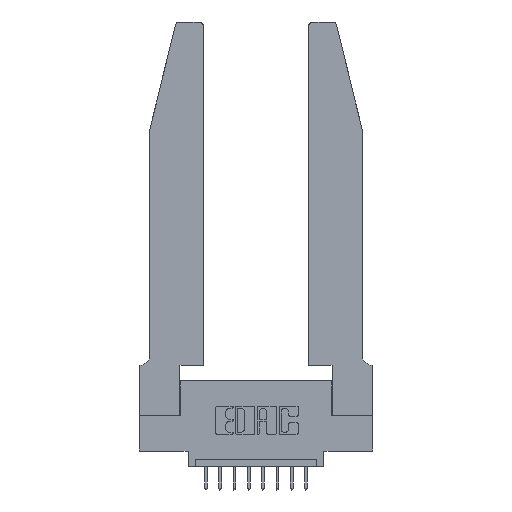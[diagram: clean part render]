
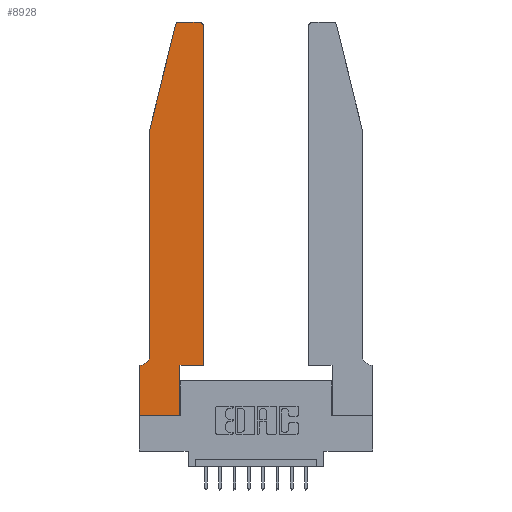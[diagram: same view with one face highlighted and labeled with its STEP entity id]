
A CAD part, top view. The second image highlights one B-rep face of the part: STEP entity #8928.
In plain terms, the highlighted planar face has unit normal (0, 0, 1).
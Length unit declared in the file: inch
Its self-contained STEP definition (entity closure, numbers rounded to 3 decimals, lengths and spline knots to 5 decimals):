
#104 = PLANE ( 'NONE',  #12794 ) ;
#188 = EDGE_CURVE ( 'NONE', #14460, #11975, #10427, .T. ) ;
#436 = EDGE_LOOP ( 'NONE', ( #5661, #9876, #15325, #4013, #3837, #6668, #12609, #13823, #14365, #1613, #8005, #14443 ) ) ;
#572 = VERTEX_POINT ( 'NONE', #828 ) ;
#698 = CARTESIAN_POINT ( 'NONE',  ( 0.4505, 0.35, 0.37 ) ) ;
#756 = DIRECTION ( 'NONE',  ( -1., 0., 0. ) ) ;
#828 = CARTESIAN_POINT ( 'NONE',  ( 0.4505, 0.35, 0.37 ) ) ;
#941 = AXIS2_PLACEMENT_3D ( 'NONE', #3066, #14900, #7694 ) ;
#1211 = CARTESIAN_POINT ( 'NONE',  ( 0., 0., 0.37 ) ) ;
#1532 = CARTESIAN_POINT ( 'NONE',  ( 0.2865, 0.35, 0.37 ) ) ;
#1562 = CARTESIAN_POINT ( 'NONE',  ( 0.0755, 0.42, 0.37 ) ) ;
#1613 = ORIENTED_EDGE ( 'NONE', *, *, #8762, .T. ) ;
#1659 = DIRECTION ( 'NONE',  ( -1., 0., 0. ) ) ;
#1669 = CARTESIAN_POINT ( 'NONE',  ( 0.0755, 0.35, 0.37 ) ) ;
#1812 = DIRECTION ( 'NONE',  ( 1., 0., 0. ) ) ;
#1844 = LINE ( 'NONE', #698, #15187 ) ;
#1859 = DIRECTION ( 'NONE',  ( 0., 1., 0. ) ) ;
#1860 = LINE ( 'NONE', #6751, #10148 ) ;
#1892 = DIRECTION ( 'NONE',  ( 0., 0., -1. ) ) ;
#1962 = CARTESIAN_POINT ( 'NONE',  ( 0.2865, 0.35, 0.37 ) ) ;
#2010 = DIRECTION ( 'NONE',  ( 0., -1., 0. ) ) ;
#2581 = DIRECTION ( 'NONE',  ( 1., 0., 0. ) ) ;
#2660 = EDGE_CURVE ( 'NONE', #9801, #9125, #14091, .T. ) ;
#3066 = CARTESIAN_POINT ( 'NONE',  ( 0.284, 2.72, 0.37 ) ) ;
#3127 = CARTESIAN_POINT ( 'NONE',  ( 0.2605, 2.75, 0.37 ) ) ;
#3391 = DIRECTION ( 'NONE',  ( 0., 0., 1. ) ) ;
#3406 = LINE ( 'NONE', #1962, #6804 ) ;
#3455 = CIRCLE ( 'NONE', #941, 0.03 ) ;
#3666 = CARTESIAN_POINT ( 'NONE',  ( 0.4505, 2.72, 0.37 ) ) ;
#3747 = CARTESIAN_POINT ( 'NONE',  ( 0.4205, 2.75, 0.37 ) ) ;
#3837 = ORIENTED_EDGE ( 'NONE', *, *, #2660, .T. ) ;
#4013 = ORIENTED_EDGE ( 'NONE', *, *, #11783, .T. ) ;
#4332 = DIRECTION ( 'NONE',  ( -0.239, -0.971, 0. ) ) ;
#4358 = VECTOR ( 'NONE', #1812, 39.37008 ) ;
#5359 = VERTEX_POINT ( 'NONE', #12533 ) ;
#5596 = EDGE_CURVE ( 'NONE', #13138, #5359, #3455, .T. ) ;
#5661 = ORIENTED_EDGE ( 'NONE', *, *, #14688, .T. ) ;
#5752 = CARTESIAN_POINT ( 'NONE',  ( 0.4205, 2.72, 0.37 ) ) ;
#5823 = CARTESIAN_POINT ( 'NONE',  ( 0.0755, 2., 0.37 ) ) ;
#6138 = AXIS2_PLACEMENT_3D ( 'NONE', #9379, #1892, #1659 ) ;
#6334 = CARTESIAN_POINT ( 'NONE',  ( 0.284, 2.75, 0.37 ) ) ;
#6430 = CARTESIAN_POINT ( 'NONE',  ( 0., 0.35, 0.37 ) ) ;
#6586 = VECTOR ( 'NONE', #13824, 39.37008 ) ;
#6668 = ORIENTED_EDGE ( 'NONE', *, *, #7223, .T. ) ;
#6709 = DIRECTION ( 'NONE',  ( 0., 1., 0. ) ) ;
#6751 = CARTESIAN_POINT ( 'NONE',  ( 0.0755, 2., 0.37 ) ) ;
#6754 = DIRECTION ( 'NONE',  ( 0., -1., 0. ) ) ;
#6804 = VECTOR ( 'NONE', #1859, 39.37008 ) ;
#6903 = DIRECTION ( 'NONE',  ( 1., 0., 0. ) ) ;
#6921 = DIRECTION ( 'NONE',  ( 1., 0., 0. ) ) ;
#7105 = LINE ( 'NONE', #7278, #13544 ) ;
#7223 = EDGE_CURVE ( 'NONE', #9125, #10531, #10176, .T. ) ;
#7278 = CARTESIAN_POINT ( 'NONE',  ( 0.4505, 0.35, 0.37 ) ) ;
#7694 = DIRECTION ( 'NONE',  ( 1., 0., 0. ) ) ;
#8005 = ORIENTED_EDGE ( 'NONE', *, *, #9090, .T. ) ;
#8097 = EDGE_CURVE ( 'NONE', #10531, #10298, #15389, .T. ) ;
#8352 = CARTESIAN_POINT ( 'NONE',  ( 0.0055, 0.35, 0.37 ) ) ;
#8762 = EDGE_CURVE ( 'NONE', #11982, #572, #1844, .T. ) ;
#8928 = ADVANCED_FACE ( 'NONE', ( #12033 ), #104, .T. ) ;
#9077 = LINE ( 'NONE', #13902, #10984 ) ;
#9090 = EDGE_CURVE ( 'NONE', #572, #14460, #7105, .T. ) ;
#9125 = VERTEX_POINT ( 'NONE', #8352 ) ;
#9343 = CARTESIAN_POINT ( 'NONE',  ( 0.2865, 0., 0.37 ) ) ;
#9379 = CARTESIAN_POINT ( 'NONE',  ( 0.0055, 0.42, 0.37 ) ) ;
#9595 = AXIS2_PLACEMENT_3D ( 'NONE', #5752, #3391, #6921 ) ;
#9801 = VERTEX_POINT ( 'NONE', #1562 ) ;
#9842 = CARTESIAN_POINT ( 'NONE',  ( 0., 0., 0.37 ) ) ;
#9876 = ORIENTED_EDGE ( 'NONE', *, *, #5596, .T. ) ;
#10148 = VECTOR ( 'NONE', #4332, 39.37008 ) ;
#10176 = LINE ( 'NONE', #1669, #6586 ) ;
#10298 = VERTEX_POINT ( 'NONE', #1211 ) ;
#10427 = CIRCLE ( 'NONE', #9595, 0.03 ) ;
#10531 = VERTEX_POINT ( 'NONE', #6430 ) ;
#10666 = VECTOR ( 'NONE', #756, 39.37008 ) ;
#10984 = VECTOR ( 'NONE', #2010, 39.37008 ) ;
#11267 = LINE ( 'NONE', #3127, #10666 ) ;
#11366 = LINE ( 'NONE', #11548, #4358 ) ;
#11448 = EDGE_CURVE ( 'NONE', #10298, #14787, #11366, .T. ) ;
#11548 = CARTESIAN_POINT ( 'NONE',  ( 0., 0., 0.37 ) ) ;
#11756 = EDGE_CURVE ( 'NONE', #14787, #11982, #3406, .T. ) ;
#11783 = EDGE_CURVE ( 'NONE', #14165, #9801, #9077, .T. ) ;
#11975 = VERTEX_POINT ( 'NONE', #3747 ) ;
#11982 = VERTEX_POINT ( 'NONE', #1532 ) ;
#12033 = FACE_OUTER_BOUND ( 'NONE', #436, .T. ) ;
#12177 = CARTESIAN_POINT ( 'NONE',  ( 0., 0.35, 0.37 ) ) ;
#12533 = CARTESIAN_POINT ( 'NONE',  ( 0.25487, 2.72718, 0.37 ) ) ;
#12609 = ORIENTED_EDGE ( 'NONE', *, *, #8097, .T. ) ;
#12794 = AXIS2_PLACEMENT_3D ( 'NONE', #12177, #13373, #2581 ) ;
#13138 = VERTEX_POINT ( 'NONE', #6334 ) ;
#13287 = EDGE_CURVE ( 'NONE', #5359, #14165, #1860, .T. ) ;
#13373 = DIRECTION ( 'NONE',  ( 0., 0., 1. ) ) ;
#13544 = VECTOR ( 'NONE', #6709, 39.37008 ) ;
#13557 = VECTOR ( 'NONE', #6754, 39.37008 ) ;
#13823 = ORIENTED_EDGE ( 'NONE', *, *, #11448, .T. ) ;
#13824 = DIRECTION ( 'NONE',  ( -1., 0., 0. ) ) ;
#13902 = CARTESIAN_POINT ( 'NONE',  ( 0.0755, 2., 0.37 ) ) ;
#14091 = CIRCLE ( 'NONE', #6138, 0.07 ) ;
#14165 = VERTEX_POINT ( 'NONE', #5823 ) ;
#14365 = ORIENTED_EDGE ( 'NONE', *, *, #11756, .T. ) ;
#14443 = ORIENTED_EDGE ( 'NONE', *, *, #188, .T. ) ;
#14460 = VERTEX_POINT ( 'NONE', #3666 ) ;
#14688 = EDGE_CURVE ( 'NONE', #11975, #13138, #11267, .T. ) ;
#14787 = VERTEX_POINT ( 'NONE', #9343 ) ;
#14900 = DIRECTION ( 'NONE',  ( 0., 0., 1. ) ) ;
#15187 = VECTOR ( 'NONE', #6903, 39.37008 ) ;
#15325 = ORIENTED_EDGE ( 'NONE', *, *, #13287, .T. ) ;
#15389 = LINE ( 'NONE', #9842, #13557 ) ;
